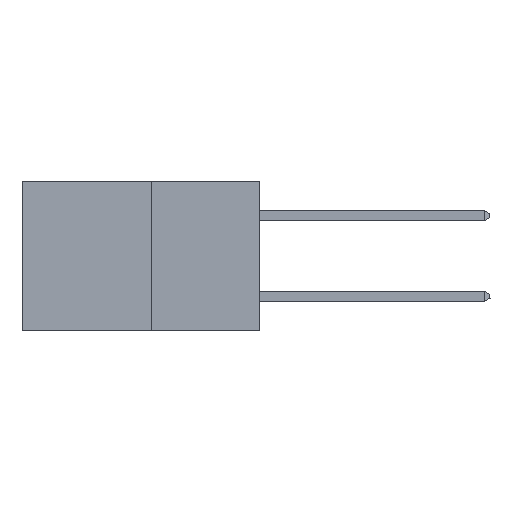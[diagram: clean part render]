
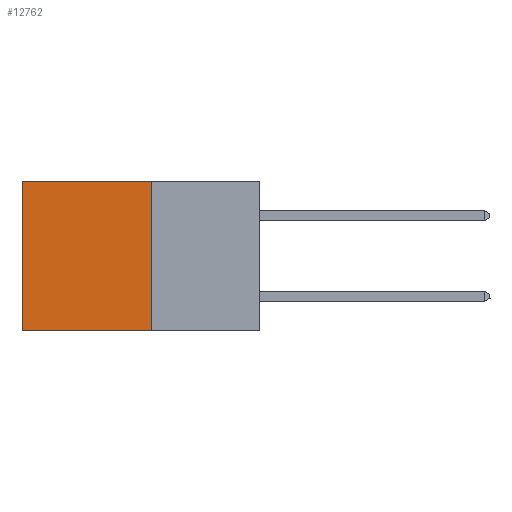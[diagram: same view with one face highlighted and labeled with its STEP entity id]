
A CAD part, left-side view. The second image highlights one B-rep face of the part: STEP entity #12762.
In plain terms, the highlighted planar face has unit normal (-1, 0, 0).
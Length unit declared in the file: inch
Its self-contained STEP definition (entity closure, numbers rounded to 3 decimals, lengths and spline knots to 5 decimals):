
#103 = VERTEX_POINT ( 'NONE', #8140 ) ;
#127 = CARTESIAN_POINT ( 'NONE',  ( 0.277, 0.59, 0. ) ) ;
#415 = VERTEX_POINT ( 'NONE', #127 ) ;
#1050 = EDGE_CURVE ( 'NONE', #103, #1420, #8898, .T. ) ;
#1420 = VERTEX_POINT ( 'NONE', #8162 ) ;
#2467 = VECTOR ( 'NONE', #5299, 39.37008 ) ;
#2478 = PLANE ( 'NONE',  #10960 ) ;
#3261 = LINE ( 'NONE', #14573, #9627 ) ;
#3629 = DIRECTION ( 'NONE',  ( 1., 0., 0. ) ) ;
#3790 = ORIENTED_EDGE ( 'NONE', *, *, #13506, .T. ) ;
#4156 = CARTESIAN_POINT ( 'NONE',  ( 0.277, 0.27, -0.37 ) ) ;
#5115 = EDGE_CURVE ( 'NONE', #10693, #415, #9231, .T. ) ;
#5299 = DIRECTION ( 'NONE',  ( 0., 0., -1. ) ) ;
#5540 = LINE ( 'NONE', #4156, #2467 ) ;
#6161 = EDGE_CURVE ( 'NONE', #10693, #103, #5540, .T. ) ;
#8104 = DIRECTION ( 'NONE',  ( 0., 0., -1. ) ) ;
#8110 = FACE_OUTER_BOUND ( 'NONE', #11852, .T. ) ;
#8140 = CARTESIAN_POINT ( 'NONE',  ( 0.277, 0.27, -0.37 ) ) ;
#8162 = CARTESIAN_POINT ( 'NONE',  ( 0.277, 0.59, -0.37 ) ) ;
#8553 = VECTOR ( 'NONE', #12048, 39.37008 ) ;
#8896 = VECTOR ( 'NONE', #12307, 39.37008 ) ;
#8898 = LINE ( 'NONE', #11473, #8553 ) ;
#9052 = ORIENTED_EDGE ( 'NONE', *, *, #1050, .F. ) ;
#9231 = LINE ( 'NONE', #13390, #8896 ) ;
#9263 = CARTESIAN_POINT ( 'NONE',  ( 0.277, 0.27, -0.37 ) ) ;
#9627 = VECTOR ( 'NONE', #8104, 39.37008 ) ;
#10212 = ORIENTED_EDGE ( 'NONE', *, *, #6161, .F. ) ;
#10693 = VERTEX_POINT ( 'NONE', #11735 ) ;
#10960 = AXIS2_PLACEMENT_3D ( 'NONE', #9263, #3629, #11423 ) ;
#11263 = ORIENTED_EDGE ( 'NONE', *, *, #5115, .T. ) ;
#11423 = DIRECTION ( 'NONE',  ( 0., 0., -1. ) ) ;
#11473 = CARTESIAN_POINT ( 'NONE',  ( 0.277, 0.27, -0.37 ) ) ;
#11735 = CARTESIAN_POINT ( 'NONE',  ( 0.277, 0.27, 0. ) ) ;
#11852 = EDGE_LOOP ( 'NONE', ( #3790, #9052, #10212, #11263 ) ) ;
#12048 = DIRECTION ( 'NONE',  ( 0., 1., 0. ) ) ;
#12307 = DIRECTION ( 'NONE',  ( 0., 1., 0. ) ) ;
#12762 = ADVANCED_FACE ( 'NONE', ( #8110 ), #2478, .F. ) ;
#13390 = CARTESIAN_POINT ( 'NONE',  ( 0.277, 0.27, 0. ) ) ;
#13506 = EDGE_CURVE ( 'NONE', #415, #1420, #3261, .T. ) ;
#14573 = CARTESIAN_POINT ( 'NONE',  ( 0.277, 0.59, -0.37 ) ) ;
